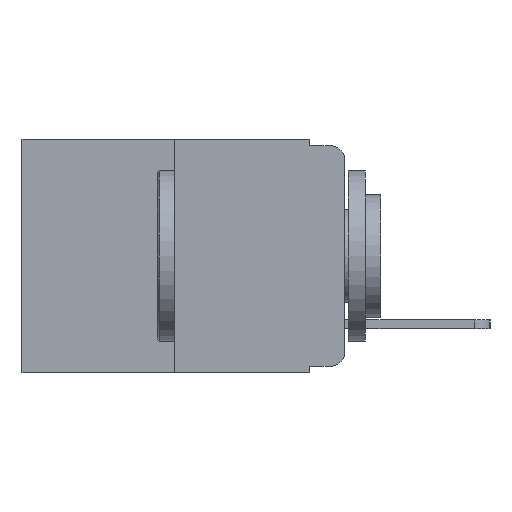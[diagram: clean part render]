
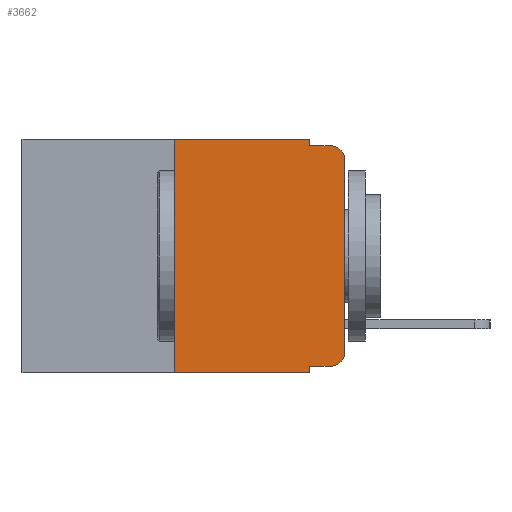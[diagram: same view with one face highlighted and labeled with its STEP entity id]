
A CAD part, left-side view. The second image highlights one B-rep face of the part: STEP entity #3662.
In plain terms, the highlighted planar face has unit normal (-1, 0, 0).
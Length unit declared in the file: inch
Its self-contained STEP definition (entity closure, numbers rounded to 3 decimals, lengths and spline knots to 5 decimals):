
#5 = VECTOR ( 'NONE', #7492, 39.37008 ) ;
#219 = ORIENTED_EDGE ( 'NONE', *, *, #14485, .F. ) ;
#268 = VERTEX_POINT ( 'NONE', #7752 ) ;
#586 = VECTOR ( 'NONE', #17341, 39.37008 ) ;
#589 = VECTOR ( 'NONE', #6521, 39.37008 ) ;
#591 = DIRECTION ( 'NONE',  ( -1., 0., 0. ) ) ;
#850 = EDGE_CURVE ( 'NONE', #11271, #268, #12702, .T. ) ;
#1743 = DIRECTION ( 'NONE',  ( 1., 0., 0. ) ) ;
#1979 = CARTESIAN_POINT ( 'NONE',  ( 0., 0., -0.313 ) ) ;
#2045 = CARTESIAN_POINT ( 'NONE',  ( 0., 0.02, -0.313 ) ) ;
#2310 = CARTESIAN_POINT ( 'NONE',  ( 0., 0.25, 0. ) ) ;
#3368 = PLANE ( 'NONE',  #17409 ) ;
#3372 = CARTESIAN_POINT ( 'NONE',  ( 0., 0.051, 0. ) ) ;
#3662 = ADVANCED_FACE ( 'NONE', ( #7176 ), #3368, .F. ) ;
#3714 = DIRECTION ( 'NONE',  ( 0., 0., -1. ) ) ;
#3743 = VERTEX_POINT ( 'NONE', #1979 ) ;
#4299 = ORIENTED_EDGE ( 'NONE', *, *, #13304, .T. ) ;
#4351 = EDGE_LOOP ( 'NONE', ( #10653, #13461, #13913, #219, #14151, #7299, #13734, #18021, #9415, #4299 ) ) ;
#4471 = EDGE_CURVE ( 'NONE', #3743, #19105, #6787, .T. ) ;
#4961 = LINE ( 'NONE', #16364, #12678 ) ;
#5443 = LINE ( 'NONE', #2310, #8946 ) ;
#5463 = CARTESIAN_POINT ( 'NONE',  ( 0., 0.051, -0.333 ) ) ;
#5837 = CARTESIAN_POINT ( 'NONE',  ( 0., 0.051, 0. ) ) ;
#6521 = DIRECTION ( 'NONE',  ( 0., -1., 0. ) ) ;
#6787 = LINE ( 'NONE', #13438, #17735 ) ;
#7068 = VECTOR ( 'NONE', #10414, 39.37008 ) ;
#7176 = FACE_OUTER_BOUND ( 'NONE', #4351, .T. ) ;
#7299 = ORIENTED_EDGE ( 'NONE', *, *, #9851, .F. ) ;
#7422 = CARTESIAN_POINT ( 'NONE',  ( 0., 0.051, 0. ) ) ;
#7492 = DIRECTION ( 'NONE',  ( 0., -1., 0. ) ) ;
#7539 = LINE ( 'NONE', #5837, #7068 ) ;
#7546 = VERTEX_POINT ( 'NONE', #17796 ) ;
#7752 = CARTESIAN_POINT ( 'NONE',  ( 0., 0.02, -0.333 ) ) ;
#7821 = AXIS2_PLACEMENT_3D ( 'NONE', #9965, #591, #11363 ) ;
#7832 = DIRECTION ( 'NONE',  ( 0., 0., 1. ) ) ;
#7917 = DIRECTION ( 'NONE',  ( 0., -1., 0. ) ) ;
#8028 = CARTESIAN_POINT ( 'NONE',  ( 0., 0.051, -0.01 ) ) ;
#8417 = AXIS2_PLACEMENT_3D ( 'NONE', #2045, #12473, #3714 ) ;
#8946 = VECTOR ( 'NONE', #14079, 39.37008 ) ;
#8971 = LINE ( 'NONE', #18852, #5 ) ;
#9391 = CARTESIAN_POINT ( 'NONE',  ( 0., 0.473, 0. ) ) ;
#9415 = ORIENTED_EDGE ( 'NONE', *, *, #850, .T. ) ;
#9518 = VERTEX_POINT ( 'NONE', #12105 ) ;
#9773 = CARTESIAN_POINT ( 'NONE',  ( 0., 0., -0.03 ) ) ;
#9851 = EDGE_CURVE ( 'NONE', #16908, #7546, #5443, .T. ) ;
#9965 = CARTESIAN_POINT ( 'NONE',  ( 0., 0.02, -0.03 ) ) ;
#10414 = DIRECTION ( 'NONE',  ( 0., 0., -1. ) ) ;
#10653 = ORIENTED_EDGE ( 'NONE', *, *, #4471, .T. ) ;
#10820 = CARTESIAN_POINT ( 'NONE',  ( 0., 0.473, 0. ) ) ;
#11271 = VERTEX_POINT ( 'NONE', #11959 ) ;
#11363 = DIRECTION ( 'NONE',  ( 0., 0., -1. ) ) ;
#11666 = LINE ( 'NONE', #9391, #14471 ) ;
#11959 = CARTESIAN_POINT ( 'NONE',  ( 0., 0.051, -0.333 ) ) ;
#12061 = EDGE_CURVE ( 'NONE', #11271, #14688, #12698, .T. ) ;
#12086 = EDGE_CURVE ( 'NONE', #16908, #14688, #8971, .T. ) ;
#12105 = CARTESIAN_POINT ( 'NONE',  ( 0., 0.02, -0.01 ) ) ;
#12248 = DIRECTION ( 'NONE',  ( 0., 0., -1. ) ) ;
#12380 = CARTESIAN_POINT ( 'NONE',  ( 0., 0.051, -0.343 ) ) ;
#12473 = DIRECTION ( 'NONE',  ( -1., 0., 0. ) ) ;
#12628 = CARTESIAN_POINT ( 'NONE',  ( 0., 0.25, -0.343 ) ) ;
#12678 = VECTOR ( 'NONE', #7917, 39.37008 ) ;
#12698 = LINE ( 'NONE', #7422, #586 ) ;
#12702 = LINE ( 'NONE', #5463, #589 ) ;
#13077 = VERTEX_POINT ( 'NONE', #3372 ) ;
#13304 = EDGE_CURVE ( 'NONE', #268, #3743, #13507, .T. ) ;
#13438 = CARTESIAN_POINT ( 'NONE',  ( 0., 0., 0. ) ) ;
#13461 = ORIENTED_EDGE ( 'NONE', *, *, #19241, .T. ) ;
#13507 = CIRCLE ( 'NONE', #8417, 0.02 ) ;
#13567 = DIRECTION ( 'NONE',  ( 0., -1., 0. ) ) ;
#13734 = ORIENTED_EDGE ( 'NONE', *, *, #12086, .T. ) ;
#13913 = ORIENTED_EDGE ( 'NONE', *, *, #15432, .F. ) ;
#14079 = DIRECTION ( 'NONE',  ( 0., 0., 1. ) ) ;
#14151 = ORIENTED_EDGE ( 'NONE', *, *, #18746, .F. ) ;
#14471 = VECTOR ( 'NONE', #13567, 39.37008 ) ;
#14485 = EDGE_CURVE ( 'NONE', #13077, #17226, #7539, .T. ) ;
#14688 = VERTEX_POINT ( 'NONE', #12380 ) ;
#15432 = EDGE_CURVE ( 'NONE', #17226, #9518, #4961, .T. ) ;
#16364 = CARTESIAN_POINT ( 'NONE',  ( 0., 0.051, -0.01 ) ) ;
#16908 = VERTEX_POINT ( 'NONE', #12628 ) ;
#17226 = VERTEX_POINT ( 'NONE', #8028 ) ;
#17341 = DIRECTION ( 'NONE',  ( 0., 0., -1. ) ) ;
#17409 = AXIS2_PLACEMENT_3D ( 'NONE', #10820, #1743, #12248 ) ;
#17735 = VECTOR ( 'NONE', #7832, 39.37008 ) ;
#17796 = CARTESIAN_POINT ( 'NONE',  ( 0., 0.25, 0. ) ) ;
#18021 = ORIENTED_EDGE ( 'NONE', *, *, #12061, .F. ) ;
#18317 = CIRCLE ( 'NONE', #7821, 0.02 ) ;
#18746 = EDGE_CURVE ( 'NONE', #7546, #13077, #11666, .T. ) ;
#18852 = CARTESIAN_POINT ( 'NONE',  ( 0., 0.473, -0.343 ) ) ;
#19105 = VERTEX_POINT ( 'NONE', #9773 ) ;
#19241 = EDGE_CURVE ( 'NONE', #19105, #9518, #18317, .T. ) ;
